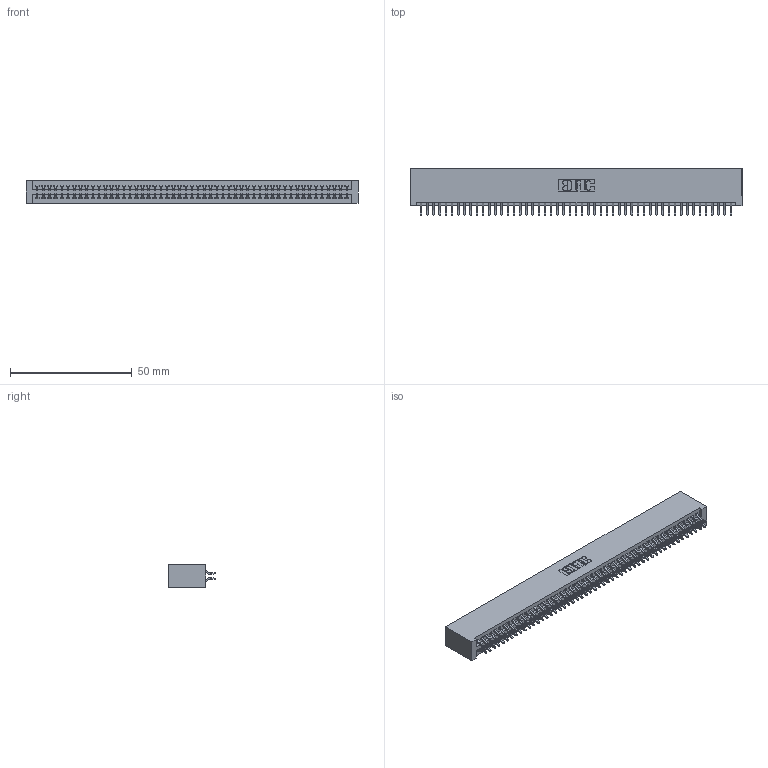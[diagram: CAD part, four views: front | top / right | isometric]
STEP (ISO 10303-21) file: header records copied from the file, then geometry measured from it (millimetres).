
FILE_DESCRIPTION (( 'STEP AP203' ), '1' );
FILE_NAME ('345-102-556-201.STEP', '2018-10-05T20:55:43', ( '' ), ( '' ), 'SwSTEP 2.0', 'SolidWorks 2016', '' );
FILE_SCHEMA (( 'CONFIG_CONTROL_DESIGN' ));
Length unit declared in the file: inch
Products named in the file (3): 345-102-556-201; 345-292-001_556 Tail; 345 Part_No Mounting Lugs
Assembly tree (103 placements, depth 2):
  345-102-556-201
    345 Part_No Mounting Lugs
    345-292-001_556 Tail  x102
Bounding box: 136.14 x 19.24 x 9.4 mm (x, y, z)
Volume: 13920.6 mm3; surface area: 20965.2 mm2
Topology: 103 solids, 103 shells, 5830 faces, 17351 edges, 11430 vertices
Faces by surface type: plane 3850, cylinder 1980
Entity records: 38747 total; most frequent: CARTESIAN_POINT 6500, ORIENTED_EDGE 6422, DIRECTION 5703, EDGE_CURVE 3211, LINE 2875, VECTOR 2875, VERTEX_POINT 2138, AXIS2_PLACEMENT_3D 1414
